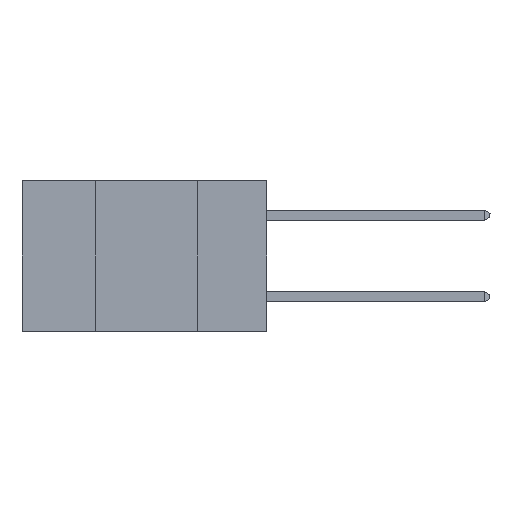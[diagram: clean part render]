
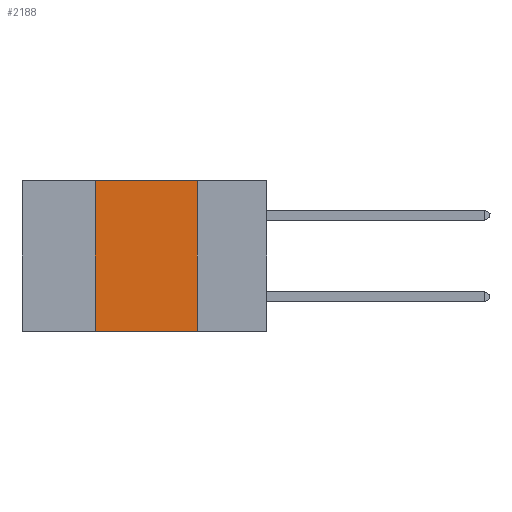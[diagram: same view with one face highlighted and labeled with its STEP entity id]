
A CAD part, left-side view. The second image highlights one B-rep face of the part: STEP entity #2188.
In plain terms, the highlighted planar face has unit normal (-1, 0, 0).
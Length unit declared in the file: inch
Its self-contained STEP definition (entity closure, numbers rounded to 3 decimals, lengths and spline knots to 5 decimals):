
#2188 = ADVANCED_FACE ( 'NONE', ( #20870 ), #4688, .F. ) ;
#2384 = ORIENTED_EDGE ( 'NONE', *, *, #15059, .T. ) ;
#2947 = LINE ( 'NONE', #16117, #31179 ) ;
#3536 = VECTOR ( 'NONE', #28041, 39.37008 ) ;
#3676 = CARTESIAN_POINT ( 'NONE',  ( 0., 0.6, -0.37 ) ) ;
#3911 = CARTESIAN_POINT ( 'NONE',  ( 0., 0.42, 0. ) ) ;
#4688 = PLANE ( 'NONE',  #9071 ) ;
#4894 = DIRECTION ( 'NONE',  ( 0., 0., -1. ) ) ;
#5699 = EDGE_CURVE ( 'NONE', #30560, #7829, #2947, .T. ) ;
#6630 = LINE ( 'NONE', #35780, #18569 ) ;
#6726 = EDGE_CURVE ( 'NONE', #7829, #9335, #6630, .T. ) ;
#6924 = LINE ( 'NONE', #3676, #11174 ) ;
#7829 = VERTEX_POINT ( 'NONE', #3911 ) ;
#8219 = CARTESIAN_POINT ( 'NONE',  ( 0., 0.17, 0. ) ) ;
#9071 = AXIS2_PLACEMENT_3D ( 'NONE', #30819, #24546, #4894 ) ;
#9335 = VERTEX_POINT ( 'NONE', #8219 ) ;
#11174 = VECTOR ( 'NONE', #16852, 39.37008 ) ;
#13946 = LINE ( 'NONE', #19997, #3536 ) ;
#15059 = EDGE_CURVE ( 'NONE', #30560, #41113, #6924, .T. ) ;
#16117 = CARTESIAN_POINT ( 'NONE',  ( 0., 0.42, 0. ) ) ;
#16348 = DIRECTION ( 'NONE',  ( 0., -1., 0. ) ) ;
#16852 = DIRECTION ( 'NONE',  ( 0., -1., 0. ) ) ;
#17156 = EDGE_CURVE ( 'NONE', #9335, #41113, #13946, .T. ) ;
#18569 = VECTOR ( 'NONE', #16348, 39.37008 ) ;
#19997 = CARTESIAN_POINT ( 'NONE',  ( 0., 0.17, 0. ) ) ;
#20870 = FACE_OUTER_BOUND ( 'NONE', #29180, .T. ) ;
#24546 = DIRECTION ( 'NONE',  ( 1., 0., 0. ) ) ;
#25077 = ORIENTED_EDGE ( 'NONE', *, *, #5699, .F. ) ;
#28041 = DIRECTION ( 'NONE',  ( 0., 0., -1. ) ) ;
#29180 = EDGE_LOOP ( 'NONE', ( #38281, #42174, #25077, #2384 ) ) ;
#29300 = DIRECTION ( 'NONE',  ( 0., 0., 1. ) ) ;
#30560 = VERTEX_POINT ( 'NONE', #41503 ) ;
#30819 = CARTESIAN_POINT ( 'NONE',  ( 0., 0.6, 0. ) ) ;
#31179 = VECTOR ( 'NONE', #29300, 39.37008 ) ;
#34476 = CARTESIAN_POINT ( 'NONE',  ( 0., 0.17, -0.37 ) ) ;
#35780 = CARTESIAN_POINT ( 'NONE',  ( 0., 0.6, 0. ) ) ;
#38281 = ORIENTED_EDGE ( 'NONE', *, *, #17156, .F. ) ;
#41113 = VERTEX_POINT ( 'NONE', #34476 ) ;
#41503 = CARTESIAN_POINT ( 'NONE',  ( 0., 0.42, -0.37 ) ) ;
#42174 = ORIENTED_EDGE ( 'NONE', *, *, #6726, .F. ) ;
